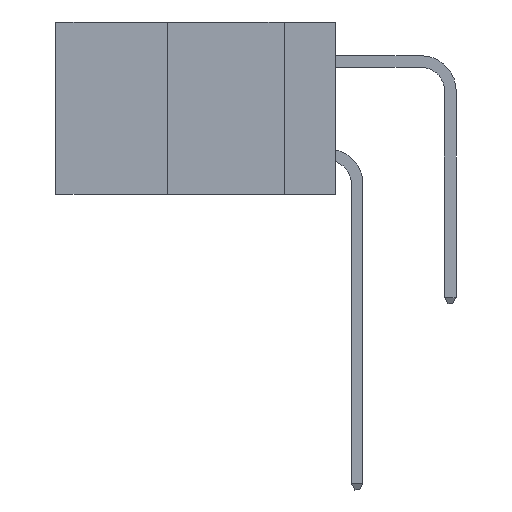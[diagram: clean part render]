
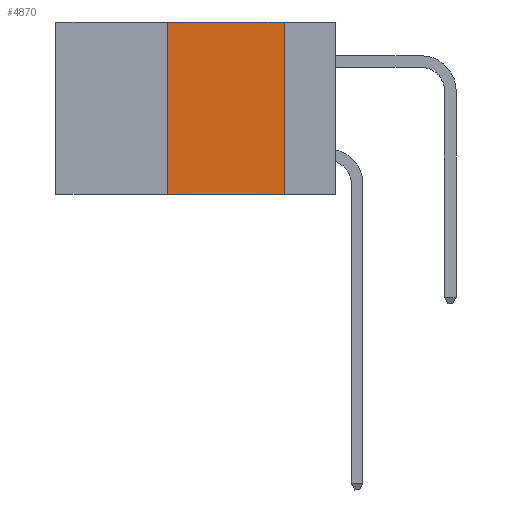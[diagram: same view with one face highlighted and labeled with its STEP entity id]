
A CAD part, left-side view. The second image highlights one B-rep face of the part: STEP entity #4870.
In plain terms, the highlighted planar face has unit normal (-1, 0, 0).
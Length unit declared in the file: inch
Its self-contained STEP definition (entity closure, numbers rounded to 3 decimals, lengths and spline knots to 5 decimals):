
#43 = VECTOR ( 'NONE', #21010, 39.37008 ) ;
#173 = EDGE_CURVE ( 'NONE', #2075, #5740, #14737, .T. ) ;
#1440 = ORIENTED_EDGE ( 'NONE', *, *, #14980, .F. ) ;
#1991 = CARTESIAN_POINT ( 'NONE',  ( 0., 0.36, 0. ) ) ;
#2028 = EDGE_CURVE ( 'NONE', #2701, #19124, #5522, .T. ) ;
#2075 = VERTEX_POINT ( 'NONE', #14425 ) ;
#2322 = FACE_OUTER_BOUND ( 'NONE', #7157, .T. ) ;
#2701 = VERTEX_POINT ( 'NONE', #1991 ) ;
#4511 = CARTESIAN_POINT ( 'NONE',  ( 0., 0.6, 0. ) ) ;
#4870 = ADVANCED_FACE ( 'NONE', ( #2322 ), #9266, .F. ) ;
#4942 = EDGE_CURVE ( 'NONE', #19124, #5740, #18830, .T. ) ;
#4967 = LINE ( 'NONE', #13005, #43 ) ;
#5522 = LINE ( 'NONE', #17776, #20783 ) ;
#5740 = VERTEX_POINT ( 'NONE', #9713 ) ;
#6504 = DIRECTION ( 'NONE',  ( 0., -1., 0. ) ) ;
#6798 = DIRECTION ( 'NONE',  ( 0., -1., 0. ) ) ;
#6817 = CARTESIAN_POINT ( 'NONE',  ( 0., 0.11, 0. ) ) ;
#7157 = EDGE_LOOP ( 'NONE', ( #19545, #7171, #1440, #12018 ) ) ;
#7171 = ORIENTED_EDGE ( 'NONE', *, *, #2028, .F. ) ;
#8231 = DIRECTION ( 'NONE',  ( 1., 0., 0. ) ) ;
#8308 = AXIS2_PLACEMENT_3D ( 'NONE', #4511, #8231, #14871 ) ;
#9266 = PLANE ( 'NONE',  #8308 ) ;
#9713 = CARTESIAN_POINT ( 'NONE',  ( 0., 0.11, -0.37 ) ) ;
#10415 = VECTOR ( 'NONE', #6798, 39.37008 ) ;
#10883 = CARTESIAN_POINT ( 'NONE',  ( 0., 0.11, 0. ) ) ;
#12018 = ORIENTED_EDGE ( 'NONE', *, *, #173, .T. ) ;
#13005 = CARTESIAN_POINT ( 'NONE',  ( 0., 0.36, 0. ) ) ;
#14425 = CARTESIAN_POINT ( 'NONE',  ( 0., 0.36, -0.37 ) ) ;
#14737 = LINE ( 'NONE', #15126, #10415 ) ;
#14871 = DIRECTION ( 'NONE',  ( 0., 0., -1. ) ) ;
#14980 = EDGE_CURVE ( 'NONE', #2075, #2701, #4967, .T. ) ;
#15126 = CARTESIAN_POINT ( 'NONE',  ( 0., 0.6, -0.37 ) ) ;
#17776 = CARTESIAN_POINT ( 'NONE',  ( 0., 0.6, 0. ) ) ;
#18184 = DIRECTION ( 'NONE',  ( 0., 0., -1. ) ) ;
#18830 = LINE ( 'NONE', #6817, #20919 ) ;
#19124 = VERTEX_POINT ( 'NONE', #10883 ) ;
#19545 = ORIENTED_EDGE ( 'NONE', *, *, #4942, .F. ) ;
#20783 = VECTOR ( 'NONE', #6504, 39.37008 ) ;
#20919 = VECTOR ( 'NONE', #18184, 39.37008 ) ;
#21010 = DIRECTION ( 'NONE',  ( 0., 0., 1. ) ) ;
